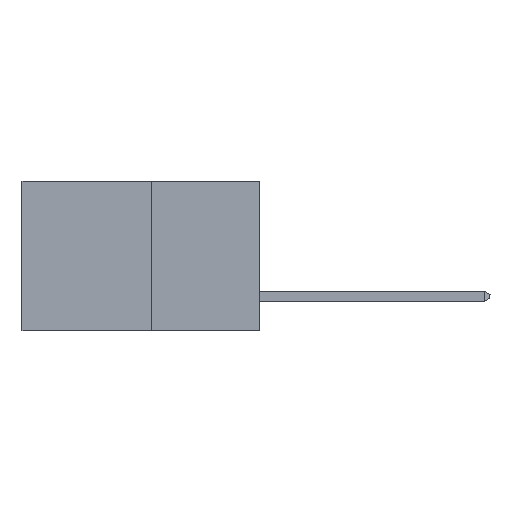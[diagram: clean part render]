
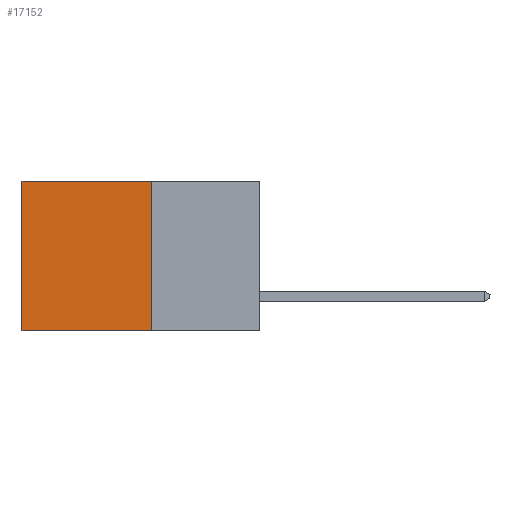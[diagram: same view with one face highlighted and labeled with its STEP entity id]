
A CAD part, left-side view. The second image highlights one B-rep face of the part: STEP entity #17152.
In plain terms, the highlighted planar face has unit normal (-1, 0, 0).
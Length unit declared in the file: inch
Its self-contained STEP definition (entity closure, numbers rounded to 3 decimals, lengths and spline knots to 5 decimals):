
#653 = CARTESIAN_POINT ( 'NONE',  ( 0.277, 0.59, -0.37 ) ) ;
#1015 = DIRECTION ( 'NONE',  ( 0., 1., 0. ) ) ;
#3074 = VECTOR ( 'NONE', #13357, 39.37008 ) ;
#3565 = DIRECTION ( 'NONE',  ( 0., 0., -1. ) ) ;
#3938 = ORIENTED_EDGE ( 'NONE', *, *, #13626, .F. ) ;
#4039 = DIRECTION ( 'NONE',  ( 0., 1., 0. ) ) ;
#5544 = VERTEX_POINT ( 'NONE', #9854 ) ;
#6092 = VERTEX_POINT ( 'NONE', #25444 ) ;
#8194 = VERTEX_POINT ( 'NONE', #10048 ) ;
#8675 = EDGE_CURVE ( 'NONE', #5544, #13519, #16136, .T. ) ;
#9773 = CARTESIAN_POINT ( 'NONE',  ( 0.277, 0.27, -0.37 ) ) ;
#9854 = CARTESIAN_POINT ( 'NONE',  ( 0.277, 0.59, 0. ) ) ;
#10048 = CARTESIAN_POINT ( 'NONE',  ( 0.277, 0.27, 0. ) ) ;
#10192 = LINE ( 'NONE', #17204, #14688 ) ;
#12007 = DIRECTION ( 'NONE',  ( 0., 0., -1. ) ) ;
#13357 = DIRECTION ( 'NONE',  ( 0., 0., -1. ) ) ;
#13519 = VERTEX_POINT ( 'NONE', #653 ) ;
#13626 = EDGE_CURVE ( 'NONE', #8194, #6092, #14764, .T. ) ;
#13898 = ORIENTED_EDGE ( 'NONE', *, *, #8675, .T. ) ;
#13978 = ORIENTED_EDGE ( 'NONE', *, *, #14240, .T. ) ;
#14161 = FACE_OUTER_BOUND ( 'NONE', #26421, .T. ) ;
#14240 = EDGE_CURVE ( 'NONE', #8194, #5544, #26136, .T. ) ;
#14483 = AXIS2_PLACEMENT_3D ( 'NONE', #27770, #16723, #3565 ) ;
#14537 = PLANE ( 'NONE',  #14483 ) ;
#14688 = VECTOR ( 'NONE', #4039, 39.37008 ) ;
#14764 = LINE ( 'NONE', #9773, #19931 ) ;
#15046 = VECTOR ( 'NONE', #1015, 39.37008 ) ;
#16136 = LINE ( 'NONE', #21107, #3074 ) ;
#16723 = DIRECTION ( 'NONE',  ( 1., 0., 0. ) ) ;
#17152 = ADVANCED_FACE ( 'NONE', ( #14161 ), #14537, .F. ) ;
#17204 = CARTESIAN_POINT ( 'NONE',  ( 0.277, 0.27, -0.37 ) ) ;
#17371 = ORIENTED_EDGE ( 'NONE', *, *, #25150, .F. ) ;
#19931 = VECTOR ( 'NONE', #12007, 39.37008 ) ;
#21107 = CARTESIAN_POINT ( 'NONE',  ( 0.277, 0.59, -0.37 ) ) ;
#25150 = EDGE_CURVE ( 'NONE', #6092, #13519, #10192, .T. ) ;
#25444 = CARTESIAN_POINT ( 'NONE',  ( 0.277, 0.27, -0.37 ) ) ;
#26136 = LINE ( 'NONE', #27424, #15046 ) ;
#26421 = EDGE_LOOP ( 'NONE', ( #13898, #17371, #3938, #13978 ) ) ;
#27424 = CARTESIAN_POINT ( 'NONE',  ( 0.277, 0.27, 0. ) ) ;
#27770 = CARTESIAN_POINT ( 'NONE',  ( 0.277, 0.27, -0.37 ) ) ;
